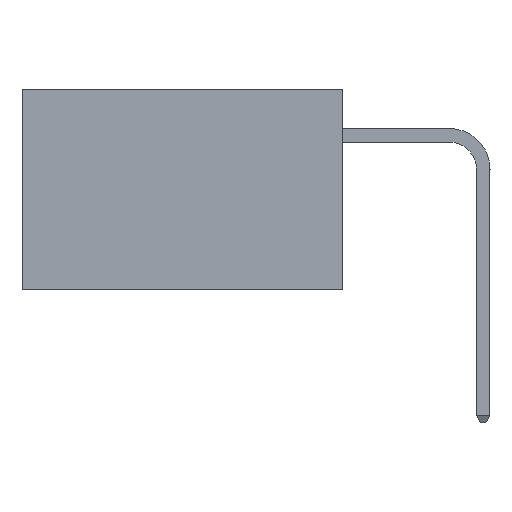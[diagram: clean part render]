
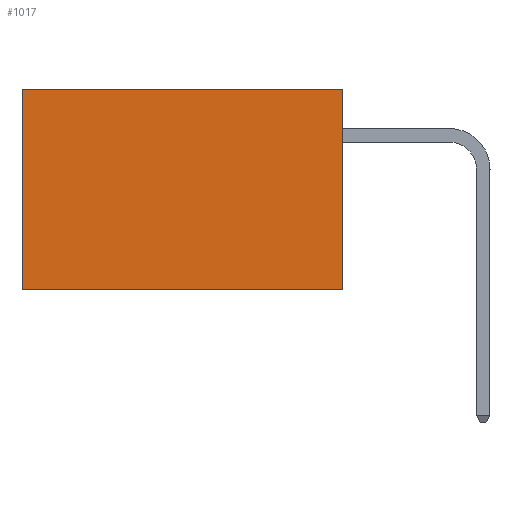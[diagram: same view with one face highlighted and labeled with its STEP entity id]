
A CAD part, left-side view. The second image highlights one B-rep face of the part: STEP entity #1017.
In plain terms, the highlighted planar face has unit normal (-1, 0, 0).
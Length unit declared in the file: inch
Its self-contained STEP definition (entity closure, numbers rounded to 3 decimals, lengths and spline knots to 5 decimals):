
#297 = VERTEX_POINT ( 'NONE', #11460 ) ;
#1017 = ADVANCED_FACE ( 'NONE', ( #4392 ), #3929, .F. ) ;
#1303 = EDGE_LOOP ( 'NONE', ( #12323, #5450, #7875, #10320 ) ) ;
#1341 = EDGE_CURVE ( 'NONE', #297, #3098, #9424, .T. ) ;
#1529 = AXIS2_PLACEMENT_3D ( 'NONE', #5394, #3489, #9898 ) ;
#1767 = VERTEX_POINT ( 'NONE', #8635 ) ;
#1836 = LINE ( 'NONE', #7707, #11455 ) ;
#2153 = LINE ( 'NONE', #3958, #6886 ) ;
#2226 = VECTOR ( 'NONE', #7871, 39.37008 ) ;
#3098 = VERTEX_POINT ( 'NONE', #5208 ) ;
#3282 = DIRECTION ( 'NONE',  ( 0., 0., -1. ) ) ;
#3424 = EDGE_CURVE ( 'NONE', #3098, #3527, #2153, .T. ) ;
#3489 = DIRECTION ( 'NONE',  ( 1., 0., 0. ) ) ;
#3527 = VERTEX_POINT ( 'NONE', #8759 ) ;
#3929 = PLANE ( 'NONE',  #1529 ) ;
#3958 = CARTESIAN_POINT ( 'NONE',  ( 0.277, 0.59, -0.37 ) ) ;
#4392 = FACE_OUTER_BOUND ( 'NONE', #1303, .T. ) ;
#5208 = CARTESIAN_POINT ( 'NONE',  ( 0.277, 0.59, 0. ) ) ;
#5394 = CARTESIAN_POINT ( 'NONE',  ( 0.277, 0., -0.37 ) ) ;
#5450 = ORIENTED_EDGE ( 'NONE', *, *, #9213, .F. ) ;
#6730 = EDGE_CURVE ( 'NONE', #297, #1767, #9557, .T. ) ;
#6886 = VECTOR ( 'NONE', #9490, 39.37008 ) ;
#7092 = VECTOR ( 'NONE', #3282, 39.37008 ) ;
#7707 = CARTESIAN_POINT ( 'NONE',  ( 0.277, 0., -0.37 ) ) ;
#7871 = DIRECTION ( 'NONE',  ( 0., 1., 0. ) ) ;
#7875 = ORIENTED_EDGE ( 'NONE', *, *, #6730, .F. ) ;
#7900 = CARTESIAN_POINT ( 'NONE',  ( 0.277, 0., -0.37 ) ) ;
#8635 = CARTESIAN_POINT ( 'NONE',  ( 0.277, 0., -0.37 ) ) ;
#8642 = DIRECTION ( 'NONE',  ( 0., 1., 0. ) ) ;
#8759 = CARTESIAN_POINT ( 'NONE',  ( 0.277, 0.59, -0.37 ) ) ;
#9213 = EDGE_CURVE ( 'NONE', #1767, #3527, #1836, .T. ) ;
#9424 = LINE ( 'NONE', #11749, #2226 ) ;
#9490 = DIRECTION ( 'NONE',  ( 0., 0., -1. ) ) ;
#9557 = LINE ( 'NONE', #7900, #7092 ) ;
#9898 = DIRECTION ( 'NONE',  ( 0., 0., -1. ) ) ;
#10320 = ORIENTED_EDGE ( 'NONE', *, *, #1341, .T. ) ;
#11455 = VECTOR ( 'NONE', #8642, 39.37008 ) ;
#11460 = CARTESIAN_POINT ( 'NONE',  ( 0.277, 0., 0. ) ) ;
#11749 = CARTESIAN_POINT ( 'NONE',  ( 0.277, 0., 0. ) ) ;
#12323 = ORIENTED_EDGE ( 'NONE', *, *, #3424, .T. ) ;
